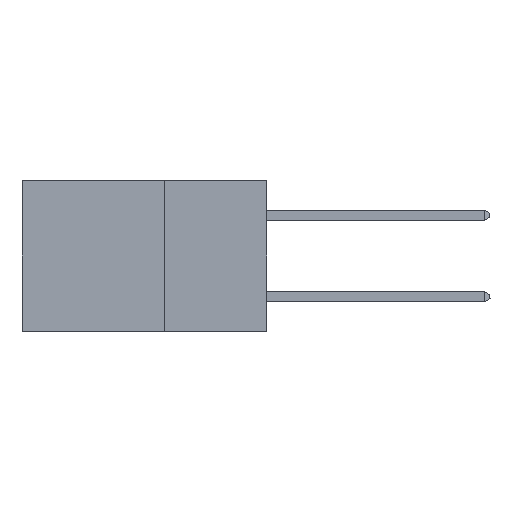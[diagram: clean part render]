
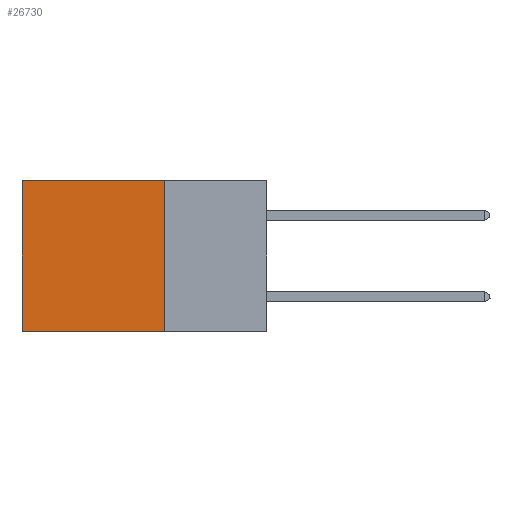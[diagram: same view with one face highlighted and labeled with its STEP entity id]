
A CAD part, left-side view. The second image highlights one B-rep face of the part: STEP entity #26730.
In plain terms, the highlighted planar face has unit normal (-1, 0, 0).
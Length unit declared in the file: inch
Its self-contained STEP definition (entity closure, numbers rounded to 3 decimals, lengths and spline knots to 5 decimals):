
#889 = DIRECTION ( 'NONE',  ( 0., 1., 0. ) ) ;
#2242 = VERTEX_POINT ( 'NONE', #17349 ) ;
#3127 = ORIENTED_EDGE ( 'NONE', *, *, #7803, .T. ) ;
#3382 = CARTESIAN_POINT ( 'NONE',  ( 0.2875, 0.6, 0. ) ) ;
#5161 = EDGE_CURVE ( 'NONE', #12370, #35409, #19487, .T. ) ;
#6362 = ORIENTED_EDGE ( 'NONE', *, *, #5161, .F. ) ;
#7803 = EDGE_CURVE ( 'NONE', #20624, #2242, #29157, .T. ) ;
#9762 = CARTESIAN_POINT ( 'NONE',  ( 0.2875, 0.25, -0.37 ) ) ;
#12370 = VERTEX_POINT ( 'NONE', #21047 ) ;
#13674 = LINE ( 'NONE', #28237, #22594 ) ;
#14832 = CARTESIAN_POINT ( 'NONE',  ( 0.2875, 0.25, 0. ) ) ;
#15895 = LINE ( 'NONE', #21017, #30634 ) ;
#16043 = FACE_OUTER_BOUND ( 'NONE', #29181, .T. ) ;
#16483 = ORIENTED_EDGE ( 'NONE', *, *, #29945, .T. ) ;
#16997 = DIRECTION ( 'NONE',  ( 0., 0., -1. ) ) ;
#17349 = CARTESIAN_POINT ( 'NONE',  ( 0.2875, 0.6, -0.37 ) ) ;
#19487 = LINE ( 'NONE', #14832, #35511 ) ;
#20624 = VERTEX_POINT ( 'NONE', #22957 ) ;
#21017 = CARTESIAN_POINT ( 'NONE',  ( 0.2875, 0.25, 0. ) ) ;
#21047 = CARTESIAN_POINT ( 'NONE',  ( 0.2875, 0.25, 0. ) ) ;
#22594 = VECTOR ( 'NONE', #31042, 39.37008 ) ;
#22957 = CARTESIAN_POINT ( 'NONE',  ( 0.2875, 0.6, 0. ) ) ;
#23552 = ORIENTED_EDGE ( 'NONE', *, *, #30382, .F. ) ;
#23715 = DIRECTION ( 'NONE',  ( 0., 0., -1. ) ) ;
#23781 = DIRECTION ( 'NONE',  ( 0., 0., -1. ) ) ;
#25743 = DIRECTION ( 'NONE',  ( 1., 0., 0. ) ) ;
#26240 = AXIS2_PLACEMENT_3D ( 'NONE', #36056, #25743, #16997 ) ;
#26730 = ADVANCED_FACE ( 'NONE', ( #16043 ), #33945, .F. ) ;
#28237 = CARTESIAN_POINT ( 'NONE',  ( 0.2875, 0.25, -0.37 ) ) ;
#29157 = LINE ( 'NONE', #3382, #36671 ) ;
#29181 = EDGE_LOOP ( 'NONE', ( #3127, #23552, #6362, #16483 ) ) ;
#29945 = EDGE_CURVE ( 'NONE', #12370, #20624, #15895, .T. ) ;
#30382 = EDGE_CURVE ( 'NONE', #35409, #2242, #13674, .T. ) ;
#30634 = VECTOR ( 'NONE', #889, 39.37008 ) ;
#31042 = DIRECTION ( 'NONE',  ( 0., 1., 0. ) ) ;
#33945 = PLANE ( 'NONE',  #26240 ) ;
#35409 = VERTEX_POINT ( 'NONE', #9762 ) ;
#35511 = VECTOR ( 'NONE', #23715, 39.37008 ) ;
#36056 = CARTESIAN_POINT ( 'NONE',  ( 0.2875, 0.25, 0. ) ) ;
#36671 = VECTOR ( 'NONE', #23781, 39.37008 ) ;
